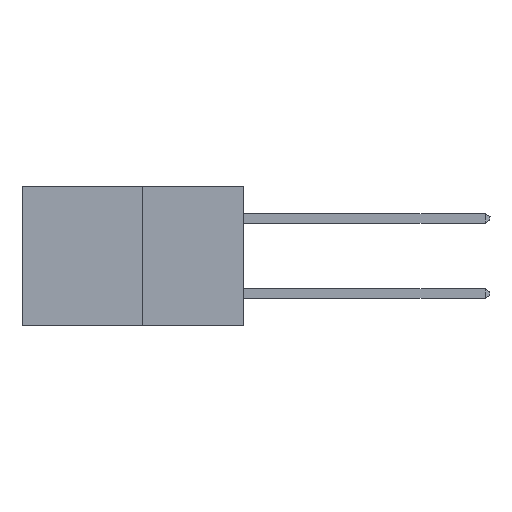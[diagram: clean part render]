
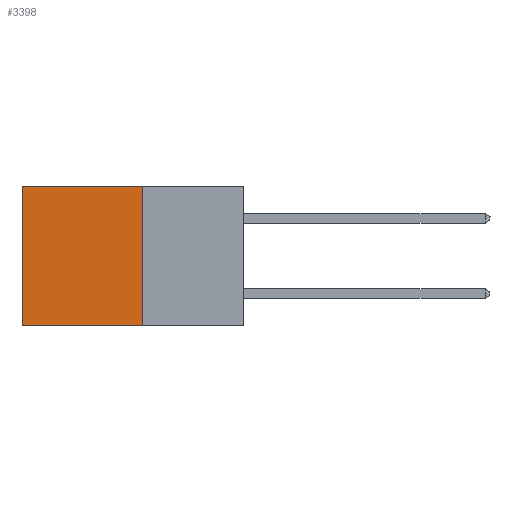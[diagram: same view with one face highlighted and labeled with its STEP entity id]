
A CAD part, left-side view. The second image highlights one B-rep face of the part: STEP entity #3398.
In plain terms, the highlighted planar face has unit normal (-1, 0, 0).
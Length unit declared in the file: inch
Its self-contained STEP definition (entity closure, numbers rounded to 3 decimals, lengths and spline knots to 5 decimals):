
#97 = EDGE_LOOP ( 'NONE', ( #735, #18829, #14725, #15342 ) ) ;
#735 = ORIENTED_EDGE ( 'NONE', *, *, #14702, .T. ) ;
#978 = CARTESIAN_POINT ( 'NONE',  ( 0.277, 0.27, -0.37 ) ) ;
#2385 = VERTEX_POINT ( 'NONE', #4340 ) ;
#3027 = DIRECTION ( 'NONE',  ( 0., 0., -1. ) ) ;
#3398 = ADVANCED_FACE ( 'NONE', ( #8061 ), #16291, .F. ) ;
#3544 = DIRECTION ( 'NONE',  ( 1., 0., 0. ) ) ;
#4010 = LINE ( 'NONE', #5547, #24052 ) ;
#4292 = CARTESIAN_POINT ( 'NONE',  ( 0.277, 0.27, 0. ) ) ;
#4340 = CARTESIAN_POINT ( 'NONE',  ( 0.277, 0.27, -0.37 ) ) ;
#5547 = CARTESIAN_POINT ( 'NONE',  ( 0.277, 0.27, 0. ) ) ;
#5947 = CARTESIAN_POINT ( 'NONE',  ( 0.277, 0.59, 0. ) ) ;
#6642 = CARTESIAN_POINT ( 'NONE',  ( 0.277, 0.27, -0.37 ) ) ;
#8061 = FACE_OUTER_BOUND ( 'NONE', #97, .T. ) ;
#10229 = EDGE_CURVE ( 'NONE', #2385, #16835, #22567, .T. ) ;
#10321 = LINE ( 'NONE', #978, #24347 ) ;
#11375 = VERTEX_POINT ( 'NONE', #4292 ) ;
#11566 = EDGE_CURVE ( 'NONE', #11375, #14522, #4010, .T. ) ;
#14198 = DIRECTION ( 'NONE',  ( 0., 0., -1. ) ) ;
#14522 = VERTEX_POINT ( 'NONE', #5947 ) ;
#14702 = EDGE_CURVE ( 'NONE', #14522, #16835, #25669, .T. ) ;
#14725 = ORIENTED_EDGE ( 'NONE', *, *, #16781, .F. ) ;
#14795 = DIRECTION ( 'NONE',  ( 0., 1., 0. ) ) ;
#15342 = ORIENTED_EDGE ( 'NONE', *, *, #11566, .T. ) ;
#15350 = CARTESIAN_POINT ( 'NONE',  ( 0.277, 0.59, -0.37 ) ) ;
#16291 = PLANE ( 'NONE',  #24862 ) ;
#16781 = EDGE_CURVE ( 'NONE', #11375, #2385, #10321, .T. ) ;
#16835 = VERTEX_POINT ( 'NONE', #15350 ) ;
#17365 = VECTOR ( 'NONE', #14795, 39.37008 ) ;
#17676 = DIRECTION ( 'NONE',  ( 0., 1., 0. ) ) ;
#18829 = ORIENTED_EDGE ( 'NONE', *, *, #10229, .F. ) ;
#18938 = CARTESIAN_POINT ( 'NONE',  ( 0.277, 0.27, -0.37 ) ) ;
#20548 = VECTOR ( 'NONE', #24431, 39.37008 ) ;
#22567 = LINE ( 'NONE', #6642, #17365 ) ;
#24052 = VECTOR ( 'NONE', #17676, 39.37008 ) ;
#24347 = VECTOR ( 'NONE', #3027, 39.37008 ) ;
#24350 = CARTESIAN_POINT ( 'NONE',  ( 0.277, 0.59, -0.37 ) ) ;
#24431 = DIRECTION ( 'NONE',  ( 0., 0., -1. ) ) ;
#24862 = AXIS2_PLACEMENT_3D ( 'NONE', #18938, #3544, #14198 ) ;
#25669 = LINE ( 'NONE', #24350, #20548 ) ;
